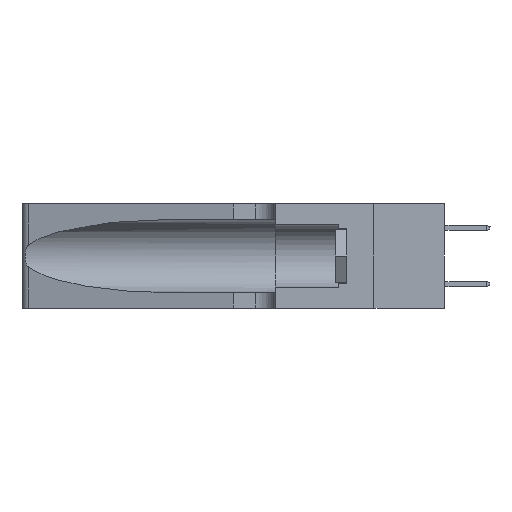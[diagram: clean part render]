
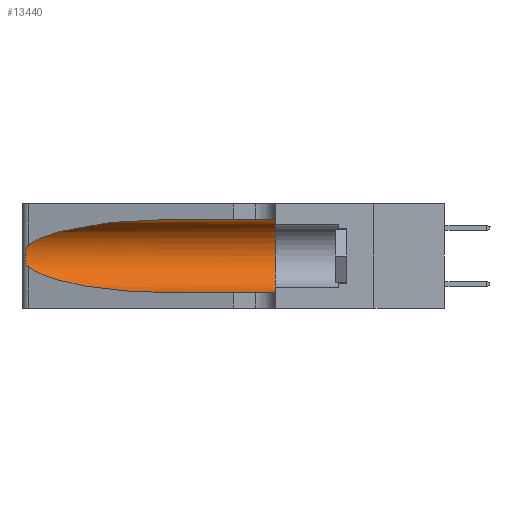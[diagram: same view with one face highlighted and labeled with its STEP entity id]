
A CAD part, left-side view. The second image highlights one B-rep face of the part: STEP entity #13440.
In plain terms, the highlighted cylindrical face has radius 3.308 mm (diameter 6.617 mm), a partial arc.
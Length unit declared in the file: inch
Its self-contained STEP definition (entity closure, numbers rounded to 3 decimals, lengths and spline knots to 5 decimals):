
#302 = CARTESIAN_POINT ( 'NONE',  ( 0.1305, 0.35, 0.31525 ) ) ;
#415 = CARTESIAN_POINT ( 'NONE',  ( 0.1305, 1.61858, 0.185 ) ) ;
#1020 = CARTESIAN_POINT ( 'NONE',  ( 0.26075, 1.23896, 0.178 ) ) ;
#2050 = CARTESIAN_POINT ( 'NONE',  ( 0.1305, 0.72297, 0.31525 ) ) ;
#2169 = ORIENTED_EDGE ( 'NONE', *, *, #5626, .T. ) ;
#2624 = CARTESIAN_POINT ( 'NONE',  ( 0.1305, 0.72297, 0.05475 ) ) ;
#2756 =( BOUNDED_CURVE ( )  B_SPLINE_CURVE ( 3, ( #4821, #13449, #22073, #8394 ),
 .UNSPECIFIED., .F., .T. ) 
 B_SPLINE_CURVE_WITH_KNOTS ( ( 4, 4 ),
 ( 3.44316, 4.71239 ),
 .UNSPECIFIED. ) 
 CURVE ( )  GEOMETRIC_REPRESENTATION_ITEM ( )  RATIONAL_B_SPLINE_CURVE ( ( 1., 0.87, 0.87, 1. ) ) 
 REPRESENTATION_ITEM ( '' )  );
#2797 = CARTESIAN_POINT ( 'NONE',  ( 0.26018, 1.23835, 0.19895 ) ) ;
#3024 = EDGE_CURVE ( 'NONE', #7092, #16721, #2756, .T. ) ;
#3757 = CARTESIAN_POINT ( 'NONE',  ( 0.2373, 1.15595, 0.28018 ) ) ;
#4506 = VERTEX_POINT ( 'NONE', #7051 ) ;
#4510 = CARTESIAN_POINT ( 'NONE',  ( 0.25789, 1.23486, 0.15765 ) ) ;
#4583 = ORIENTED_EDGE ( 'NONE', *, *, #12071, .F. ) ;
#4606 = VERTEX_POINT ( 'NONE', #5847 ) ;
#4749 = CARTESIAN_POINT ( 'NONE',  ( 0.25487, 1.22718, 0.22369 ) ) ;
#4821 = CARTESIAN_POINT ( 'NONE',  ( 0.25487, 1.22718, 0.14631 ) ) ;
#5133 = VECTOR ( 'NONE', #16617, 39.37008 ) ;
#5205 = CYLINDRICAL_SURFACE ( 'NONE', #13744, 0.13025 ) ;
#5416 = EDGE_LOOP ( 'NONE', ( #17016, #5872, #7430, #2169, #4583, #16120 ) ) ;
#5469 = CARTESIAN_POINT ( 'NONE',  ( 0.25487, 1.22718, 0.22369 ) ) ;
#5626 = EDGE_CURVE ( 'NONE', #16721, #4506, #6244, .T. ) ;
#5847 = CARTESIAN_POINT ( 'NONE',  ( 0.1305, 0.72297, 0.31525 ) ) ;
#5872 = ORIENTED_EDGE ( 'NONE', *, *, #16161, .T. ) ;
#6092 = CARTESIAN_POINT ( 'NONE',  ( 0.25787, 1.23484, 0.2124 ) ) ;
#6244 = LINE ( 'NONE', #9346, #21799 ) ;
#6314 = CARTESIAN_POINT ( 'NONE',  ( 0.25854, 1.2359, 0.20912 ) ) ;
#7051 = CARTESIAN_POINT ( 'NONE',  ( 0.1305, 0.35, 0.05475 ) ) ;
#7092 = VERTEX_POINT ( 'NONE', #9949 ) ;
#7257 = DIRECTION ( 'NONE',  ( 0., -1., 0. ) ) ;
#7430 = ORIENTED_EDGE ( 'NONE', *, *, #3024, .T. ) ;
#8394 = CARTESIAN_POINT ( 'NONE',  ( 0.1305, 0.72297, 0.05475 ) ) ;
#8622 = LINE ( 'NONE', #21803, #5133 ) ;
#9346 = CARTESIAN_POINT ( 'NONE',  ( 0.1305, 1.61858, 0.05475 ) ) ;
#9650 = CARTESIAN_POINT ( 'NONE',  ( 0.25856, 1.23593, 0.16098 ) ) ;
#9723 = CARTESIAN_POINT ( 'NONE',  ( 0.25639, 1.23184, 0.21858 ) ) ;
#9949 = CARTESIAN_POINT ( 'NONE',  ( 0.25487, 1.22718, 0.14631 ) ) ;
#11666 =( BOUNDED_CURVE ( )  B_SPLINE_CURVE ( 3, ( #2050, #19298, #3757, #5469 ),
 .UNSPECIFIED., .F., .T. ) 
 B_SPLINE_CURVE_WITH_KNOTS ( ( 4, 4 ),
 ( 1.5708, 2.84003 ),
 .UNSPECIFIED. ) 
 CURVE ( )  GEOMETRIC_REPRESENTATION_ITEM ( )  RATIONAL_B_SPLINE_CURVE ( ( 1., 0.87, 0.87, 1. ) ) 
 REPRESENTATION_ITEM ( '' )  );
#12071 = EDGE_CURVE ( 'NONE', #14795, #4506, #20070, .T. ) ;
#13147 = CARTESIAN_POINT ( 'NONE',  ( 0.26075, 1.23896, 0.19203 ) ) ;
#13155 = EDGE_CURVE ( 'NONE', #4606, #20370, #11666, .T. ) ;
#13289 = CARTESIAN_POINT ( 'NONE',  ( 0.26017, 1.23833, 0.17102 ) ) ;
#13440 = ADVANCED_FACE ( 'NONE', ( #14603 ), #5205, .F. ) ;
#13447 = AXIS2_PLACEMENT_3D ( 'NONE', #16608, #20093, #14983 ) ;
#13449 = CARTESIAN_POINT ( 'NONE',  ( 0.2373, 1.15595, 0.08982 ) ) ;
#13744 = AXIS2_PLACEMENT_3D ( 'NONE', #415, #7257, #21172 ) ;
#14603 = FACE_OUTER_BOUND ( 'NONE', #5416, .T. ) ;
#14628 = DIRECTION ( 'NONE',  ( 0., -1., 0. ) ) ;
#14739 = B_SPLINE_CURVE_WITH_KNOTS ( 'NONE', 3,
 ( #16569, #18377, #9723, #6092, #6314, #2797, #13147, #1020, #13289, #9650, #4510, #14866, #21836, #16490 ),
 .UNSPECIFIED., .F., .F.,
 ( 4, 2, 2, 2, 2, 2, 4 ),
 ( 0., 0.00027, 0.00053, 0.00107, 0.0016, 0.00187, 0.00214 ),
 .UNSPECIFIED. ) ;
#14795 = VERTEX_POINT ( 'NONE', #302 ) ;
#14866 = CARTESIAN_POINT ( 'NONE',  ( 0.25639, 1.23186, 0.15144 ) ) ;
#14983 = DIRECTION ( 'NONE',  ( 0., 0., 1. ) ) ;
#16120 = ORIENTED_EDGE ( 'NONE', *, *, #16842, .F. ) ;
#16161 = EDGE_CURVE ( 'NONE', #20370, #7092, #14739, .T. ) ;
#16490 = CARTESIAN_POINT ( 'NONE',  ( 0.25487, 1.22718, 0.14631 ) ) ;
#16569 = CARTESIAN_POINT ( 'NONE',  ( 0.25487, 1.22718, 0.22369 ) ) ;
#16608 = CARTESIAN_POINT ( 'NONE',  ( 0.1305, 0.35, 0.185 ) ) ;
#16617 = DIRECTION ( 'NONE',  ( 0., -1., 0. ) ) ;
#16721 = VERTEX_POINT ( 'NONE', #2624 ) ;
#16842 = EDGE_CURVE ( 'NONE', #4606, #14795, #8622, .T. ) ;
#17016 = ORIENTED_EDGE ( 'NONE', *, *, #13155, .T. ) ;
#18377 = CARTESIAN_POINT ( 'NONE',  ( 0.25555, 1.22994, 0.2215 ) ) ;
#19298 = CARTESIAN_POINT ( 'NONE',  ( 0.18966, 0.96281, 0.31525 ) ) ;
#20070 = CIRCLE ( 'NONE', #13447, 0.13025 ) ;
#20093 = DIRECTION ( 'NONE',  ( 0., 1., 0. ) ) ;
#20370 = VERTEX_POINT ( 'NONE', #4749 ) ;
#21172 = DIRECTION ( 'NONE',  ( 0., 0., -1. ) ) ;
#21799 = VECTOR ( 'NONE', #14628, 39.37008 ) ;
#21803 = CARTESIAN_POINT ( 'NONE',  ( 0.1305, 1.61858, 0.31525 ) ) ;
#21836 = CARTESIAN_POINT ( 'NONE',  ( 0.25555, 1.22993, 0.14849 ) ) ;
#22073 = CARTESIAN_POINT ( 'NONE',  ( 0.18966, 0.96281, 0.05475 ) ) ;
